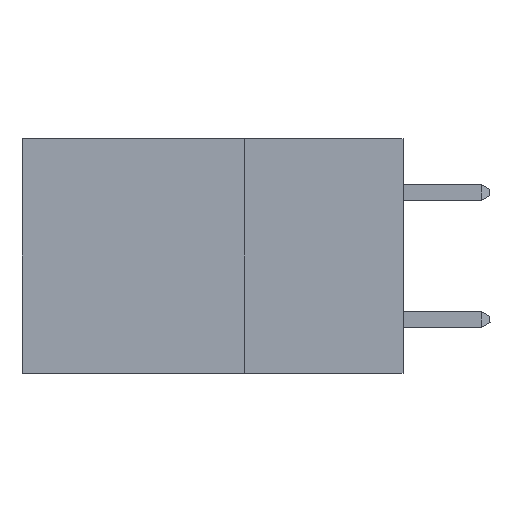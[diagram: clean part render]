
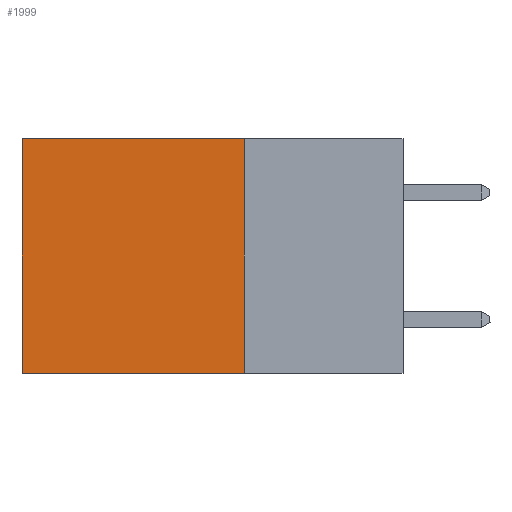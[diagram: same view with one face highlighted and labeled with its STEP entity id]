
A CAD part, left-side view. The second image highlights one B-rep face of the part: STEP entity #1999.
In plain terms, the highlighted planar face has unit normal (-1, 0, 0).
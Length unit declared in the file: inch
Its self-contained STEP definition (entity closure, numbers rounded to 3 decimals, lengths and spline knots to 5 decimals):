
#772 = DIRECTION ( 'NONE',  ( 0., 1., 0. ) ) ;
#899 = DIRECTION ( 'NONE',  ( 0., 0., -1. ) ) ;
#1988 = DIRECTION ( 'NONE',  ( 0., 0., -1. ) ) ;
#1999 = ADVANCED_FACE ( 'NONE', ( #14705 ), #3263, .F. ) ;
#2642 = VECTOR ( 'NONE', #8235, 39.37008 ) ;
#2848 = CARTESIAN_POINT ( 'NONE',  ( 0.2875, 0.25, 0. ) ) ;
#3239 = CARTESIAN_POINT ( 'NONE',  ( 0.2875, 0.6, -0.37 ) ) ;
#3263 = PLANE ( 'NONE',  #7289 ) ;
#3694 = EDGE_CURVE ( 'NONE', #15595, #4836, #4786, .T. ) ;
#4573 = EDGE_CURVE ( 'NONE', #4836, #11459, #13214, .T. ) ;
#4576 = DIRECTION ( 'NONE',  ( 0., 1., 0. ) ) ;
#4786 = LINE ( 'NONE', #7075, #2642 ) ;
#4836 = VERTEX_POINT ( 'NONE', #5811 ) ;
#5074 = ORIENTED_EDGE ( 'NONE', *, *, #4573, .F. ) ;
#5256 = LINE ( 'NONE', #9021, #14941 ) ;
#5811 = CARTESIAN_POINT ( 'NONE',  ( 0.2875, 0.25, -0.37 ) ) ;
#5973 = CARTESIAN_POINT ( 'NONE',  ( 0.2875, 0.25, 0. ) ) ;
#6623 = LINE ( 'NONE', #5973, #9594 ) ;
#7075 = CARTESIAN_POINT ( 'NONE',  ( 0.2875, 0.25, 0. ) ) ;
#7269 = ORIENTED_EDGE ( 'NONE', *, *, #3694, .F. ) ;
#7289 = AXIS2_PLACEMENT_3D ( 'NONE', #11707, #16246, #1988 ) ;
#8066 = VERTEX_POINT ( 'NONE', #11009 ) ;
#8235 = DIRECTION ( 'NONE',  ( 0., 0., -1. ) ) ;
#8901 = CARTESIAN_POINT ( 'NONE',  ( 0.2875, 0.25, -0.37 ) ) ;
#9021 = CARTESIAN_POINT ( 'NONE',  ( 0.2875, 0.6, 0. ) ) ;
#9369 = ORIENTED_EDGE ( 'NONE', *, *, #14237, .T. ) ;
#9594 = VECTOR ( 'NONE', #4576, 39.37008 ) ;
#9694 = ORIENTED_EDGE ( 'NONE', *, *, #16573, .T. ) ;
#10927 = EDGE_LOOP ( 'NONE', ( #9694, #5074, #7269, #9369 ) ) ;
#11009 = CARTESIAN_POINT ( 'NONE',  ( 0.2875, 0.6, 0. ) ) ;
#11459 = VERTEX_POINT ( 'NONE', #3239 ) ;
#11707 = CARTESIAN_POINT ( 'NONE',  ( 0.2875, 0.25, 0. ) ) ;
#12362 = VECTOR ( 'NONE', #772, 39.37008 ) ;
#13214 = LINE ( 'NONE', #8901, #12362 ) ;
#14237 = EDGE_CURVE ( 'NONE', #15595, #8066, #6623, .T. ) ;
#14705 = FACE_OUTER_BOUND ( 'NONE', #10927, .T. ) ;
#14941 = VECTOR ( 'NONE', #899, 39.37008 ) ;
#15595 = VERTEX_POINT ( 'NONE', #2848 ) ;
#16246 = DIRECTION ( 'NONE',  ( 1., 0., 0. ) ) ;
#16573 = EDGE_CURVE ( 'NONE', #8066, #11459, #5256, .T. ) ;
